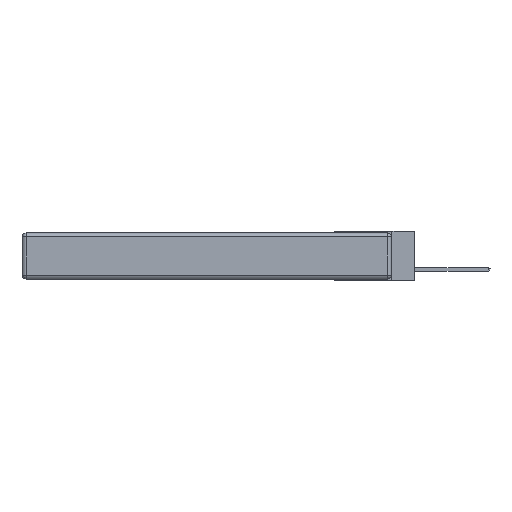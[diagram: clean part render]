
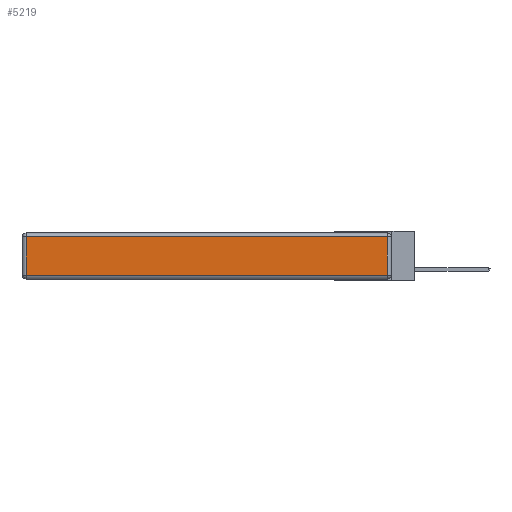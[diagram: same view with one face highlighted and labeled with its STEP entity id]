
A CAD part, left-side view. The second image highlights one B-rep face of the part: STEP entity #5219.
In plain terms, the highlighted planar face has unit normal (-1, 0, 0).
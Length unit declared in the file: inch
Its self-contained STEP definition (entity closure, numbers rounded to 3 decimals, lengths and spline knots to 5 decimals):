
#6 = DIRECTION ( 'NONE',  ( 0., -1., 0. ) ) ;
#395 = LINE ( 'NONE', #2385, #11063 ) ;
#518 = DIRECTION ( 'NONE',  ( -1., 0., 0. ) ) ;
#1014 = EDGE_CURVE ( 'NONE', #7452, #7996, #1251, .T. ) ;
#1251 = LINE ( 'NONE', #5202, #7598 ) ;
#1310 = DIRECTION ( 'NONE',  ( 0., 0., -1. ) ) ;
#1784 = VERTEX_POINT ( 'NONE', #7648 ) ;
#2385 = CARTESIAN_POINT ( 'NONE',  ( 0., 0., -0.313 ) ) ;
#3101 = DIRECTION ( 'NONE',  ( 0., 1., 0. ) ) ;
#3138 = ORIENTED_EDGE ( 'NONE', *, *, #1014, .T. ) ;
#4625 = CARTESIAN_POINT ( 'NONE',  ( 0., 2.72, -0.03 ) ) ;
#5090 = CARTESIAN_POINT ( 'NONE',  ( 0., 0.03, -0.343 ) ) ;
#5154 = VECTOR ( 'NONE', #15155, 39.37008 ) ;
#5202 = CARTESIAN_POINT ( 'NONE',  ( 0., 2.72, -0.343 ) ) ;
#5219 = ADVANCED_FACE ( 'NONE', ( #8964 ), #14407, .T. ) ;
#5444 = CARTESIAN_POINT ( 'NONE',  ( 0., 0., -0.343 ) ) ;
#6368 = CARTESIAN_POINT ( 'NONE',  ( 0., 2.72, -0.313 ) ) ;
#6436 = ORIENTED_EDGE ( 'NONE', *, *, #7321, .T. ) ;
#6803 = CARTESIAN_POINT ( 'NONE',  ( 0., 2.75, -0.03 ) ) ;
#7321 = EDGE_CURVE ( 'NONE', #11763, #1784, #12412, .T. ) ;
#7452 = VERTEX_POINT ( 'NONE', #4625 ) ;
#7493 = AXIS2_PLACEMENT_3D ( 'NONE', #5444, #518, #8928 ) ;
#7598 = VECTOR ( 'NONE', #1310, 39.37008 ) ;
#7648 = CARTESIAN_POINT ( 'NONE',  ( 0., 0.03, -0.03 ) ) ;
#7996 = VERTEX_POINT ( 'NONE', #6368 ) ;
#8819 = EDGE_LOOP ( 'NONE', ( #13931, #6436, #14954, #3138 ) ) ;
#8928 = DIRECTION ( 'NONE',  ( 0., 0., 1. ) ) ;
#8964 = FACE_OUTER_BOUND ( 'NONE', #8819, .T. ) ;
#11063 = VECTOR ( 'NONE', #6, 39.37008 ) ;
#11763 = VERTEX_POINT ( 'NONE', #12238 ) ;
#12238 = CARTESIAN_POINT ( 'NONE',  ( 0., 0.03, -0.313 ) ) ;
#12412 = LINE ( 'NONE', #5090, #5154 ) ;
#13931 = ORIENTED_EDGE ( 'NONE', *, *, #15829, .T. ) ;
#13998 = VECTOR ( 'NONE', #3101, 39.37008 ) ;
#14382 = EDGE_CURVE ( 'NONE', #1784, #7452, #15570, .T. ) ;
#14407 = PLANE ( 'NONE',  #7493 ) ;
#14954 = ORIENTED_EDGE ( 'NONE', *, *, #14382, .T. ) ;
#15155 = DIRECTION ( 'NONE',  ( 0., 0., 1. ) ) ;
#15570 = LINE ( 'NONE', #6803, #13998 ) ;
#15829 = EDGE_CURVE ( 'NONE', #7996, #11763, #395, .T. ) ;
